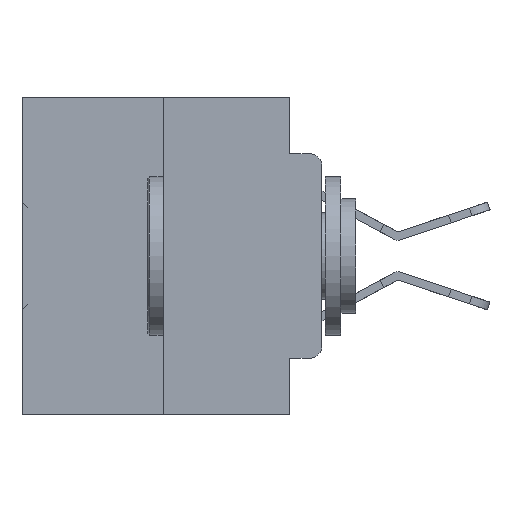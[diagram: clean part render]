
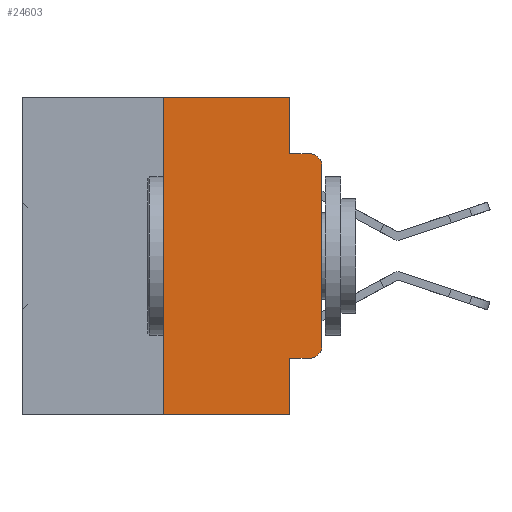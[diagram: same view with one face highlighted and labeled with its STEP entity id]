
A CAD part, left-side view. The second image highlights one B-rep face of the part: STEP entity #24603.
In plain terms, the highlighted planar face has unit normal (-1, 0, 0).
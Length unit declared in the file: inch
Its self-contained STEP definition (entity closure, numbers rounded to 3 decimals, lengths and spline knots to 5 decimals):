
#300 = DIRECTION ( 'NONE',  ( 0., 0., -1. ) ) ;
#326 = VERTEX_POINT ( 'NONE', #30767 ) ;
#613 = VERTEX_POINT ( 'NONE', #33036 ) ;
#838 = EDGE_LOOP ( 'NONE', ( #8947, #16129, #17750, #36897, #15246, #25268, #15421, #6991, #5039, #12522 ) ) ;
#993 = AXIS2_PLACEMENT_3D ( 'NONE', #24210, #9895, #21508 ) ;
#1161 = DIRECTION ( 'NONE',  ( 0., -1., 0. ) ) ;
#2071 = CARTESIAN_POINT ( 'NONE',  ( 0., 0.02, -0.0885 ) ) ;
#2336 = CARTESIAN_POINT ( 'NONE',  ( 0., 0.25, -0.5 ) ) ;
#2750 = CARTESIAN_POINT ( 'NONE',  ( 0., 0.051, 0. ) ) ;
#2824 = LINE ( 'NONE', #15342, #9642 ) ;
#2925 = VECTOR ( 'NONE', #28840, 39.37008 ) ;
#3739 = DIRECTION ( 'NONE',  ( 0., 0., 1. ) ) ;
#4446 = CARTESIAN_POINT ( 'NONE',  ( 0., 0.051, -0.0885 ) ) ;
#5039 = ORIENTED_EDGE ( 'NONE', *, *, #31321, .T. ) ;
#5995 = VECTOR ( 'NONE', #8255, 39.37008 ) ;
#6991 = ORIENTED_EDGE ( 'NONE', *, *, #37575, .F. ) ;
#8166 = EDGE_CURVE ( 'NONE', #20409, #25426, #2824, .T. ) ;
#8255 = DIRECTION ( 'NONE',  ( 0., 0., 1. ) ) ;
#8587 = PLANE ( 'NONE',  #9797 ) ;
#8784 = VECTOR ( 'NONE', #12577, 39.37008 ) ;
#8934 = VECTOR ( 'NONE', #1161, 39.37008 ) ;
#8947 = ORIENTED_EDGE ( 'NONE', *, *, #9465, .T. ) ;
#9307 = FACE_OUTER_BOUND ( 'NONE', #838, .T. ) ;
#9465 = EDGE_CURVE ( 'NONE', #37754, #17803, #14440, .T. ) ;
#9642 = VECTOR ( 'NONE', #3739, 39.37008 ) ;
#9797 = AXIS2_PLACEMENT_3D ( 'NONE', #37590, #21115, #20927 ) ;
#9895 = DIRECTION ( 'NONE',  ( -1., 0., 0. ) ) ;
#12522 = ORIENTED_EDGE ( 'NONE', *, *, #25418, .T. ) ;
#12577 = DIRECTION ( 'NONE',  ( 0., -1., 0. ) ) ;
#13540 = CARTESIAN_POINT ( 'NONE',  ( 0., 0.02, -0.4115 ) ) ;
#13916 = CARTESIAN_POINT ( 'NONE',  ( 0., 0.051, 0. ) ) ;
#14440 = LINE ( 'NONE', #34748, #5995 ) ;
#15246 = ORIENTED_EDGE ( 'NONE', *, *, #30921, .F. ) ;
#15319 = LINE ( 'NONE', #20949, #37942 ) ;
#15342 = CARTESIAN_POINT ( 'NONE',  ( 0., 0.25, 0. ) ) ;
#15421 = ORIENTED_EDGE ( 'NONE', *, *, #18813, .T. ) ;
#15853 = VERTEX_POINT ( 'NONE', #13540 ) ;
#16129 = ORIENTED_EDGE ( 'NONE', *, *, #36401, .T. ) ;
#17461 = DIRECTION ( 'NONE',  ( 0., -1., 0. ) ) ;
#17645 = VERTEX_POINT ( 'NONE', #2071 ) ;
#17750 = ORIENTED_EDGE ( 'NONE', *, *, #20789, .F. ) ;
#17803 = VERTEX_POINT ( 'NONE', #32977 ) ;
#18065 = CARTESIAN_POINT ( 'NONE',  ( 0., 0.051, -0.0885 ) ) ;
#18203 = CARTESIAN_POINT ( 'NONE',  ( 0., 0.473, 0. ) ) ;
#18813 = EDGE_CURVE ( 'NONE', #20409, #30575, #15319, .T. ) ;
#19374 = LINE ( 'NONE', #13916, #28925 ) ;
#20409 = VERTEX_POINT ( 'NONE', #2336 ) ;
#20789 = EDGE_CURVE ( 'NONE', #34015, #17645, #28017, .T. ) ;
#20927 = DIRECTION ( 'NONE',  ( 0., 0., -1. ) ) ;
#20949 = CARTESIAN_POINT ( 'NONE',  ( 0., 0.473, -0.5 ) ) ;
#20959 = AXIS2_PLACEMENT_3D ( 'NONE', #23718, #29509, #300 ) ;
#21115 = DIRECTION ( 'NONE',  ( 1., 0., 0. ) ) ;
#21508 = DIRECTION ( 'NONE',  ( 0., 0., -1. ) ) ;
#22205 = CIRCLE ( 'NONE', #20959, 0.02 ) ;
#23718 = CARTESIAN_POINT ( 'NONE',  ( 0., 0.02, -0.3915 ) ) ;
#23809 = DIRECTION ( 'NONE',  ( 0., -1., 0. ) ) ;
#24210 = CARTESIAN_POINT ( 'NONE',  ( 0., 0.02, -0.1085 ) ) ;
#24603 = ADVANCED_FACE ( 'NONE', ( #9307 ), #8587, .F. ) ;
#24913 = EDGE_CURVE ( 'NONE', #613, #34015, #19374, .T. ) ;
#25268 = ORIENTED_EDGE ( 'NONE', *, *, #8166, .F. ) ;
#25418 = EDGE_CURVE ( 'NONE', #15853, #37754, #22205, .T. ) ;
#25426 = VERTEX_POINT ( 'NONE', #26616 ) ;
#25579 = VECTOR ( 'NONE', #23809, 39.37008 ) ;
#25709 = DIRECTION ( 'NONE',  ( 0., 0., -1. ) ) ;
#25956 = LINE ( 'NONE', #2750, #2925 ) ;
#26616 = CARTESIAN_POINT ( 'NONE',  ( 0., 0.25, 0. ) ) ;
#28017 = LINE ( 'NONE', #4446, #8934 ) ;
#28840 = DIRECTION ( 'NONE',  ( 0., 0., -1. ) ) ;
#28925 = VECTOR ( 'NONE', #25709, 39.37008 ) ;
#29509 = DIRECTION ( 'NONE',  ( -1., 0., 0. ) ) ;
#29830 = CARTESIAN_POINT ( 'NONE',  ( 0., 0.051, -0.5 ) ) ;
#30189 = CARTESIAN_POINT ( 'NONE',  ( 0., 0., -0.3915 ) ) ;
#30575 = VERTEX_POINT ( 'NONE', #29830 ) ;
#30767 = CARTESIAN_POINT ( 'NONE',  ( 0., 0.051, -0.4115 ) ) ;
#30921 = EDGE_CURVE ( 'NONE', #25426, #613, #35789, .T. ) ;
#31321 = EDGE_CURVE ( 'NONE', #326, #15853, #33461, .T. ) ;
#32977 = CARTESIAN_POINT ( 'NONE',  ( 0., 0., -0.1085 ) ) ;
#33036 = CARTESIAN_POINT ( 'NONE',  ( 0., 0.051, 0. ) ) ;
#33461 = LINE ( 'NONE', #35780, #8784 ) ;
#33708 = CIRCLE ( 'NONE', #993, 0.02 ) ;
#34015 = VERTEX_POINT ( 'NONE', #18065 ) ;
#34748 = CARTESIAN_POINT ( 'NONE',  ( 0., 0., 0. ) ) ;
#35780 = CARTESIAN_POINT ( 'NONE',  ( 0., 0.051, -0.4115 ) ) ;
#35789 = LINE ( 'NONE', #18203, #25579 ) ;
#36401 = EDGE_CURVE ( 'NONE', #17803, #17645, #33708, .T. ) ;
#36897 = ORIENTED_EDGE ( 'NONE', *, *, #24913, .F. ) ;
#37575 = EDGE_CURVE ( 'NONE', #326, #30575, #25956, .T. ) ;
#37590 = CARTESIAN_POINT ( 'NONE',  ( 0., 0.473, 0. ) ) ;
#37754 = VERTEX_POINT ( 'NONE', #30189 ) ;
#37942 = VECTOR ( 'NONE', #17461, 39.37008 ) ;
